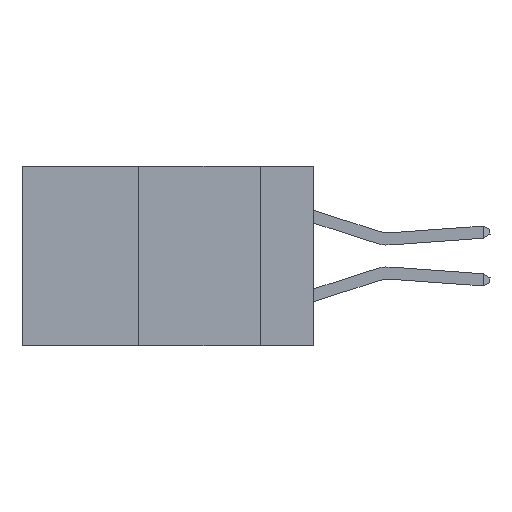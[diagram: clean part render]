
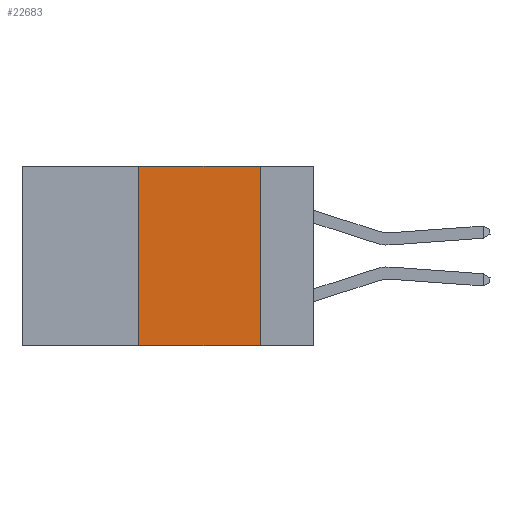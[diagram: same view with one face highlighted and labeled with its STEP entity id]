
A CAD part, left-side view. The second image highlights one B-rep face of the part: STEP entity #22683.
In plain terms, the highlighted planar face has unit normal (-1, 0, 0).
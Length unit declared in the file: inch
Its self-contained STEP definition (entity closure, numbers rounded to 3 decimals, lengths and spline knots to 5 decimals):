
#1060 = CARTESIAN_POINT ( 'NONE',  ( 0., 0.36, -0.37 ) ) ;
#1380 = LINE ( 'NONE', #19211, #8483 ) ;
#1568 = ORIENTED_EDGE ( 'NONE', *, *, #3998, .F. ) ;
#1704 = CARTESIAN_POINT ( 'NONE',  ( 0., 0.11, 0. ) ) ;
#2443 = LINE ( 'NONE', #5110, #19799 ) ;
#3998 = EDGE_CURVE ( 'NONE', #18619, #16665, #12356, .T. ) ;
#4545 = ORIENTED_EDGE ( 'NONE', *, *, #15153, .F. ) ;
#4824 = DIRECTION ( 'NONE',  ( 0., -1., 0. ) ) ;
#5110 = CARTESIAN_POINT ( 'NONE',  ( 0., 0.36, 0. ) ) ;
#6218 = FACE_OUTER_BOUND ( 'NONE', #15205, .T. ) ;
#6899 = CARTESIAN_POINT ( 'NONE',  ( 0., 0.11, 0. ) ) ;
#6901 = DIRECTION ( 'NONE',  ( 0., 0., 1. ) ) ;
#7557 = CARTESIAN_POINT ( 'NONE',  ( 0., 0.11, -0.37 ) ) ;
#7706 = ORIENTED_EDGE ( 'NONE', *, *, #9660, .F. ) ;
#7974 = AXIS2_PLACEMENT_3D ( 'NONE', #8719, #22619, #11873 ) ;
#8447 = DIRECTION ( 'NONE',  ( 0., -1., 0. ) ) ;
#8483 = VECTOR ( 'NONE', #4824, 39.37008 ) ;
#8599 = CARTESIAN_POINT ( 'NONE',  ( 0., 0.6, -0.37 ) ) ;
#8719 = CARTESIAN_POINT ( 'NONE',  ( 0., 0.6, 0. ) ) ;
#8740 = CARTESIAN_POINT ( 'NONE',  ( 0., 0.36, 0. ) ) ;
#9256 = LINE ( 'NONE', #8599, #10101 ) ;
#9660 = EDGE_CURVE ( 'NONE', #22170, #20656, #2443, .T. ) ;
#10101 = VECTOR ( 'NONE', #8447, 39.37008 ) ;
#11873 = DIRECTION ( 'NONE',  ( 0., 0., -1. ) ) ;
#12356 = LINE ( 'NONE', #6899, #18496 ) ;
#13344 = ORIENTED_EDGE ( 'NONE', *, *, #15960, .T. ) ;
#13351 = PLANE ( 'NONE',  #7974 ) ;
#14243 = DIRECTION ( 'NONE',  ( 0., 0., -1. ) ) ;
#15153 = EDGE_CURVE ( 'NONE', #20656, #18619, #1380, .T. ) ;
#15205 = EDGE_LOOP ( 'NONE', ( #1568, #4545, #7706, #13344 ) ) ;
#15960 = EDGE_CURVE ( 'NONE', #22170, #16665, #9256, .T. ) ;
#16665 = VERTEX_POINT ( 'NONE', #7557 ) ;
#18496 = VECTOR ( 'NONE', #14243, 39.37008 ) ;
#18619 = VERTEX_POINT ( 'NONE', #1704 ) ;
#19211 = CARTESIAN_POINT ( 'NONE',  ( 0., 0.6, 0. ) ) ;
#19799 = VECTOR ( 'NONE', #6901, 39.37008 ) ;
#20656 = VERTEX_POINT ( 'NONE', #8740 ) ;
#22170 = VERTEX_POINT ( 'NONE', #1060 ) ;
#22619 = DIRECTION ( 'NONE',  ( 1., 0., 0. ) ) ;
#22683 = ADVANCED_FACE ( 'NONE', ( #6218 ), #13351, .F. ) ;
